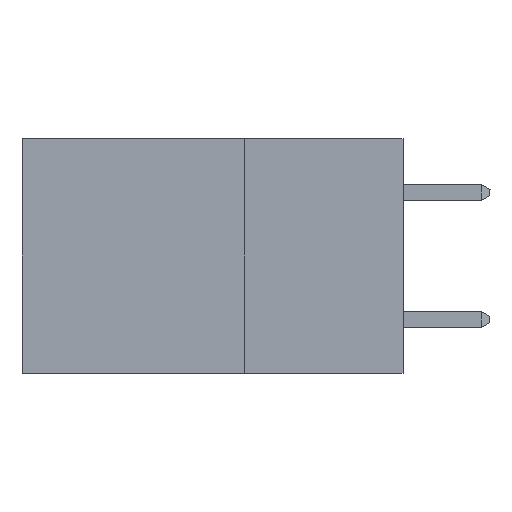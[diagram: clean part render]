
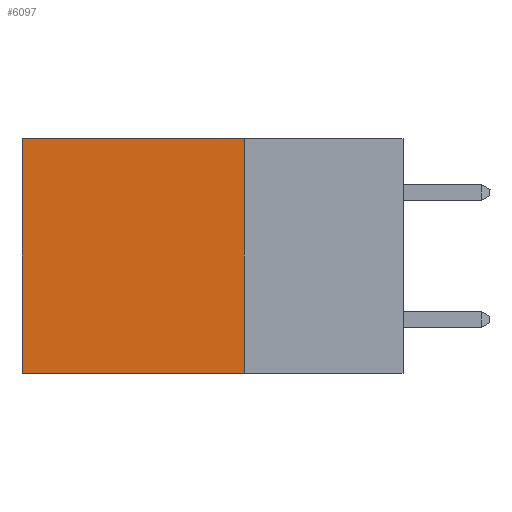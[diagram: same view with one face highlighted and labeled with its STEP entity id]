
A CAD part, left-side view. The second image highlights one B-rep face of the part: STEP entity #6097.
In plain terms, the highlighted planar face has unit normal (-1, 0, 0).
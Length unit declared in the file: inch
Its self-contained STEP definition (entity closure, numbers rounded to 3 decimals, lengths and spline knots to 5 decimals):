
#95 = VERTEX_POINT ( 'NONE', #9766 ) ;
#210 = DIRECTION ( 'NONE',  ( 0., 0., -1. ) ) ;
#1008 = ORIENTED_EDGE ( 'NONE', *, *, #7482, .F. ) ;
#1083 = VECTOR ( 'NONE', #8045, 39.37008 ) ;
#1251 = ORIENTED_EDGE ( 'NONE', *, *, #11383, .T. ) ;
#1700 = DIRECTION ( 'NONE',  ( 1., 0., 0. ) ) ;
#2323 = VERTEX_POINT ( 'NONE', #2460 ) ;
#2460 = CARTESIAN_POINT ( 'NONE',  ( 0.2875, 0.25, -0.37 ) ) ;
#2705 = FACE_OUTER_BOUND ( 'NONE', #7884, .T. ) ;
#2834 = CARTESIAN_POINT ( 'NONE',  ( 0.2875, 0.25, -0.37 ) ) ;
#2901 = LINE ( 'NONE', #5827, #7427 ) ;
#3745 = DIRECTION ( 'NONE',  ( 0., 1., 0. ) ) ;
#4195 = VERTEX_POINT ( 'NONE', #8222 ) ;
#4261 = ORIENTED_EDGE ( 'NONE', *, *, #4829, .T. ) ;
#4829 = EDGE_CURVE ( 'NONE', #4195, #8628, #8399, .T. ) ;
#5816 = ORIENTED_EDGE ( 'NONE', *, *, #9885, .F. ) ;
#5827 = CARTESIAN_POINT ( 'NONE',  ( 0.2875, 0.25, 0. ) ) ;
#6025 = VECTOR ( 'NONE', #7554, 39.37008 ) ;
#6097 = ADVANCED_FACE ( 'NONE', ( #2705 ), #8903, .F. ) ;
#7178 = CARTESIAN_POINT ( 'NONE',  ( 0.2875, 0.25, 0. ) ) ;
#7427 = VECTOR ( 'NONE', #210, 39.37008 ) ;
#7482 = EDGE_CURVE ( 'NONE', #2323, #95, #10602, .T. ) ;
#7554 = DIRECTION ( 'NONE',  ( 0., 1., 0. ) ) ;
#7876 = AXIS2_PLACEMENT_3D ( 'NONE', #10507, #1700, #8058 ) ;
#7884 = EDGE_LOOP ( 'NONE', ( #1251, #1008, #5816, #4261 ) ) ;
#8045 = DIRECTION ( 'NONE',  ( 0., 0., -1. ) ) ;
#8058 = DIRECTION ( 'NONE',  ( 0., 0., -1. ) ) ;
#8222 = CARTESIAN_POINT ( 'NONE',  ( 0.2875, 0.25, 0. ) ) ;
#8391 = LINE ( 'NONE', #8932, #1083 ) ;
#8399 = LINE ( 'NONE', #7178, #6025 ) ;
#8628 = VERTEX_POINT ( 'NONE', #9080 ) ;
#8903 = PLANE ( 'NONE',  #7876 ) ;
#8932 = CARTESIAN_POINT ( 'NONE',  ( 0.2875, 0.6, 0. ) ) ;
#8990 = VECTOR ( 'NONE', #3745, 39.37008 ) ;
#9080 = CARTESIAN_POINT ( 'NONE',  ( 0.2875, 0.6, 0. ) ) ;
#9766 = CARTESIAN_POINT ( 'NONE',  ( 0.2875, 0.6, -0.37 ) ) ;
#9885 = EDGE_CURVE ( 'NONE', #4195, #2323, #2901, .T. ) ;
#10507 = CARTESIAN_POINT ( 'NONE',  ( 0.2875, 0.25, 0. ) ) ;
#10602 = LINE ( 'NONE', #2834, #8990 ) ;
#11383 = EDGE_CURVE ( 'NONE', #8628, #95, #8391, .T. ) ;
